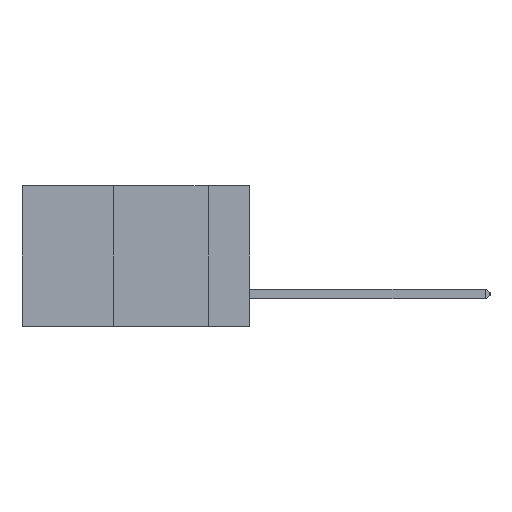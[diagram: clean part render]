
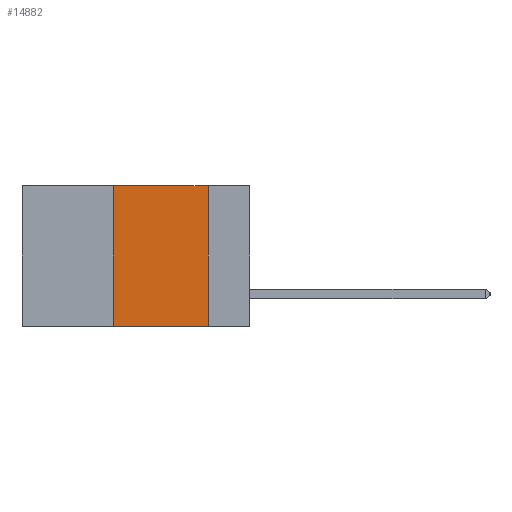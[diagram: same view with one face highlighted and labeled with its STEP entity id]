
A CAD part, left-side view. The second image highlights one B-rep face of the part: STEP entity #14882.
In plain terms, the highlighted planar face has unit normal (-1, 0, 0).
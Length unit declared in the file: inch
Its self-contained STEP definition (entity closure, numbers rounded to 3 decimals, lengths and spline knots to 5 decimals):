
#330 = DIRECTION ( 'NONE',  ( 0., 0., -1. ) ) ;
#443 = DIRECTION ( 'NONE',  ( 0., -1., 0. ) ) ;
#1437 = ORIENTED_EDGE ( 'NONE', *, *, #12243, .T. ) ;
#1784 = LINE ( 'NONE', #7944, #9865 ) ;
#1854 = LINE ( 'NONE', #8180, #17341 ) ;
#3639 = DIRECTION ( 'NONE',  ( 0., 0., 1. ) ) ;
#3780 = ORIENTED_EDGE ( 'NONE', *, *, #12511, .F. ) ;
#4468 = ORIENTED_EDGE ( 'NONE', *, *, #8447, .F. ) ;
#4557 = CARTESIAN_POINT ( 'NONE',  ( 0., 0.6, 0. ) ) ;
#4640 = VERTEX_POINT ( 'NONE', #8115 ) ;
#6604 = EDGE_CURVE ( 'NONE', #11402, #15345, #1854, .T. ) ;
#7676 = DIRECTION ( 'NONE',  ( 0., 0., -1. ) ) ;
#7894 = VERTEX_POINT ( 'NONE', #9825 ) ;
#7944 = CARTESIAN_POINT ( 'NONE',  ( 0., 0.11, 0. ) ) ;
#8115 = CARTESIAN_POINT ( 'NONE',  ( 0., 0.11, -0.37 ) ) ;
#8180 = CARTESIAN_POINT ( 'NONE',  ( 0., 0.36, 0. ) ) ;
#8447 = EDGE_CURVE ( 'NONE', #15345, #7894, #10816, .T. ) ;
#8561 = CARTESIAN_POINT ( 'NONE',  ( 0., 0.6, -0.37 ) ) ;
#9608 = AXIS2_PLACEMENT_3D ( 'NONE', #4557, #16579, #7676 ) ;
#9798 = FACE_OUTER_BOUND ( 'NONE', #15601, .T. ) ;
#9825 = CARTESIAN_POINT ( 'NONE',  ( 0., 0.11, 0. ) ) ;
#9865 = VECTOR ( 'NONE', #330, 39.37008 ) ;
#10816 = LINE ( 'NONE', #12561, #18219 ) ;
#11402 = VERTEX_POINT ( 'NONE', #14072 ) ;
#11485 = DIRECTION ( 'NONE',  ( 0., -1., 0. ) ) ;
#12243 = EDGE_CURVE ( 'NONE', #11402, #4640, #19329, .T. ) ;
#12511 = EDGE_CURVE ( 'NONE', #7894, #4640, #1784, .T. ) ;
#12561 = CARTESIAN_POINT ( 'NONE',  ( 0., 0.6, 0. ) ) ;
#13635 = PLANE ( 'NONE',  #9608 ) ;
#14072 = CARTESIAN_POINT ( 'NONE',  ( 0., 0.36, -0.37 ) ) ;
#14626 = CARTESIAN_POINT ( 'NONE',  ( 0., 0.36, 0. ) ) ;
#14882 = ADVANCED_FACE ( 'NONE', ( #9798 ), #13635, .F. ) ;
#15345 = VERTEX_POINT ( 'NONE', #14626 ) ;
#15601 = EDGE_LOOP ( 'NONE', ( #3780, #4468, #17131, #1437 ) ) ;
#16579 = DIRECTION ( 'NONE',  ( 1., 0., 0. ) ) ;
#17131 = ORIENTED_EDGE ( 'NONE', *, *, #6604, .F. ) ;
#17341 = VECTOR ( 'NONE', #3639, 39.37008 ) ;
#18219 = VECTOR ( 'NONE', #443, 39.37008 ) ;
#18894 = VECTOR ( 'NONE', #11485, 39.37008 ) ;
#19329 = LINE ( 'NONE', #8561, #18894 ) ;
